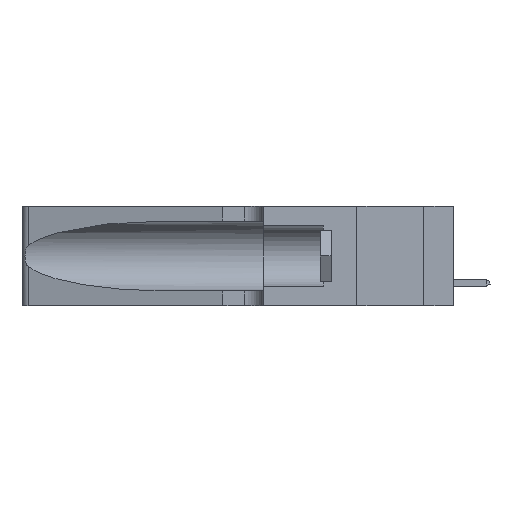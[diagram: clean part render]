
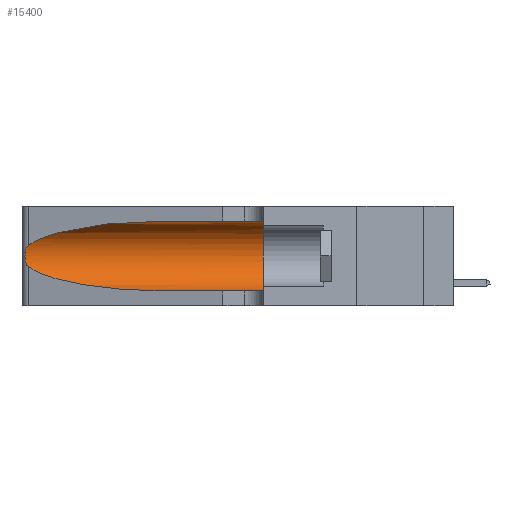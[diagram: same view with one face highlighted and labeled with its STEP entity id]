
A CAD part, left-side view. The second image highlights one B-rep face of the part: STEP entity #15400.
In plain terms, the highlighted cylindrical face has radius 3.308 mm (diameter 6.617 mm), a partial arc.
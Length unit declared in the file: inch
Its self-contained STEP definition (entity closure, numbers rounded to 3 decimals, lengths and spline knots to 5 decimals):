
#1205 = CARTESIAN_POINT ( 'NONE',  ( 0.25555, 1.22993, 0.14849 ) ) ;
#2419 = CARTESIAN_POINT ( 'NONE',  ( 0.1305, 1.61858, 0.05475 ) ) ;
#2559 = CARTESIAN_POINT ( 'NONE',  ( 0.25555, 1.22994, 0.2215 ) ) ;
#2878 = CARTESIAN_POINT ( 'NONE',  ( 0.1305, 0.35, 0.05475 ) ) ;
#3361 = EDGE_CURVE ( 'NONE', #26104, #41641, #37861, .T. ) ;
#3594 = CARTESIAN_POINT ( 'NONE',  ( 0.25639, 1.23184, 0.21858 ) ) ;
#3711 = ORIENTED_EDGE ( 'NONE', *, *, #20999, .T. ) ;
#3788 = CARTESIAN_POINT ( 'NONE',  ( 0.25854, 1.2359, 0.20912 ) ) ;
#4258 = DIRECTION ( 'NONE',  ( 0., -1., 0. ) ) ;
#4418 = CARTESIAN_POINT ( 'NONE',  ( 0.25487, 1.22718, 0.22369 ) ) ;
#4607 = CARTESIAN_POINT ( 'NONE',  ( 0.26075, 1.23896, 0.178 ) ) ;
#5104 = CARTESIAN_POINT ( 'NONE',  ( 0.26017, 1.23833, 0.17102 ) ) ;
#6530 =( BOUNDED_CURVE ( )  B_SPLINE_CURVE ( 3, ( #37726, #37422, #37571, #16501 ),
 .UNSPECIFIED., .F., .F. ) 
 B_SPLINE_CURVE_WITH_KNOTS ( ( 4, 4 ),
 ( 1.5708, 2.84003 ),
 .UNSPECIFIED. ) 
 CURVE ( )  GEOMETRIC_REPRESENTATION_ITEM ( )  RATIONAL_B_SPLINE_CURVE ( ( 1., 0.87, 0.87, 1. ) ) 
 REPRESENTATION_ITEM ( '' )  );
#10303 = CARTESIAN_POINT ( 'NONE',  ( 0.25856, 1.23593, 0.16098 ) ) ;
#10444 = CARTESIAN_POINT ( 'NONE',  ( 0.25639, 1.23186, 0.15144 ) ) ;
#12180 = EDGE_CURVE ( 'NONE', #22906, #26104, #22976, .T. ) ;
#13411 = VERTEX_POINT ( 'NONE', #21064 ) ;
#14017 = CARTESIAN_POINT ( 'NONE',  ( 0.25487, 1.22718, 0.14631 ) ) ;
#15400 = ADVANCED_FACE ( 'NONE', ( #46196 ), #45642, .F. ) ;
#15630 = ORIENTED_EDGE ( 'NONE', *, *, #21340, .T. ) ;
#16501 = CARTESIAN_POINT ( 'NONE',  ( 0.25487, 1.22718, 0.22369 ) ) ;
#16768 = ORIENTED_EDGE ( 'NONE', *, *, #12180, .F. ) ;
#18507 = CARTESIAN_POINT ( 'NONE',  ( 0.26018, 1.23835, 0.19895 ) ) ;
#19169 = CARTESIAN_POINT ( 'NONE',  ( 0.2373, 1.15595, 0.08982 ) ) ;
#20054 = CARTESIAN_POINT ( 'NONE',  ( 0.1305, 0.72297, 0.05475 ) ) ;
#20795 = DIRECTION ( 'NONE',  ( 0., -1., 0. ) ) ;
#20999 = EDGE_CURVE ( 'NONE', #25474, #33984, #41200, .T. ) ;
#21064 = CARTESIAN_POINT ( 'NONE',  ( 0.25487, 1.22718, 0.22369 ) ) ;
#21340 = EDGE_CURVE ( 'NONE', #13411, #25474, #46062, .T. ) ;
#21607 = CARTESIAN_POINT ( 'NONE',  ( 0.1305, 0.35, 0.185 ) ) ;
#21784 = EDGE_LOOP ( 'NONE', ( #43271, #15630, #3711, #34955, #45794, #16768 ) ) ;
#22006 = VECTOR ( 'NONE', #20795, 39.37008 ) ;
#22906 = VERTEX_POINT ( 'NONE', #33989 ) ;
#22976 = LINE ( 'NONE', #27740, #26335 ) ;
#23672 = CARTESIAN_POINT ( 'NONE',  ( 0.25787, 1.23484, 0.2124 ) ) ;
#25474 = VERTEX_POINT ( 'NONE', #29177 ) ;
#25748 = DIRECTION ( 'NONE',  ( 0., 0., 1. ) ) ;
#25834 = DIRECTION ( 'NONE',  ( 0., 0., -1. ) ) ;
#26016 = CARTESIAN_POINT ( 'NONE',  ( 0.18966, 0.96281, 0.05475 ) ) ;
#26104 = VERTEX_POINT ( 'NONE', #40741 ) ;
#26335 = VECTOR ( 'NONE', #30013, 39.37008 ) ;
#27740 = CARTESIAN_POINT ( 'NONE',  ( 0.1305, 1.61858, 0.31525 ) ) ;
#29007 = CARTESIAN_POINT ( 'NONE',  ( 0.1305, 1.61858, 0.185 ) ) ;
#29177 = CARTESIAN_POINT ( 'NONE',  ( 0.25487, 1.22718, 0.14631 ) ) ;
#29417 = EDGE_CURVE ( 'NONE', #33984, #41641, #30432, .T. ) ;
#29469 = CARTESIAN_POINT ( 'NONE',  ( 0.1305, 0.72297, 0.05475 ) ) ;
#30013 = DIRECTION ( 'NONE',  ( 0., -1., 0. ) ) ;
#30432 = LINE ( 'NONE', #2419, #22006 ) ;
#30737 = AXIS2_PLACEMENT_3D ( 'NONE', #29007, #4258, #25834 ) ;
#32545 = DIRECTION ( 'NONE',  ( 0., 1., 0. ) ) ;
#33984 = VERTEX_POINT ( 'NONE', #20054 ) ;
#33989 = CARTESIAN_POINT ( 'NONE',  ( 0.1305, 0.72297, 0.31525 ) ) ;
#34955 = ORIENTED_EDGE ( 'NONE', *, *, #29417, .T. ) ;
#37422 = CARTESIAN_POINT ( 'NONE',  ( 0.18966, 0.96281, 0.31525 ) ) ;
#37571 = CARTESIAN_POINT ( 'NONE',  ( 0.2373, 1.15595, 0.28018 ) ) ;
#37726 = CARTESIAN_POINT ( 'NONE',  ( 0.1305, 0.72297, 0.31525 ) ) ;
#37861 = CIRCLE ( 'NONE', #44473, 0.13025 ) ;
#40079 = CARTESIAN_POINT ( 'NONE',  ( 0.25487, 1.22718, 0.14631 ) ) ;
#40741 = CARTESIAN_POINT ( 'NONE',  ( 0.1305, 0.35, 0.31525 ) ) ;
#41200 =( BOUNDED_CURVE ( )  B_SPLINE_CURVE ( 3, ( #40079, #19169, #26016, #29469 ),
 .UNSPECIFIED., .F., .F. ) 
 B_SPLINE_CURVE_WITH_KNOTS ( ( 4, 4 ),
 ( 3.44316, 4.71239 ),
 .UNSPECIFIED. ) 
 CURVE ( )  GEOMETRIC_REPRESENTATION_ITEM ( )  RATIONAL_B_SPLINE_CURVE ( ( 1., 0.87, 0.87, 1. ) ) 
 REPRESENTATION_ITEM ( '' )  );
#41641 = VERTEX_POINT ( 'NONE', #2878 ) ;
#43271 = ORIENTED_EDGE ( 'NONE', *, *, #44158, .T. ) ;
#43517 = CARTESIAN_POINT ( 'NONE',  ( 0.26075, 1.23896, 0.19203 ) ) ;
#44158 = EDGE_CURVE ( 'NONE', #22906, #13411, #6530, .T. ) ;
#44473 = AXIS2_PLACEMENT_3D ( 'NONE', #21607, #32545, #25748 ) ;
#45642 = CYLINDRICAL_SURFACE ( 'NONE', #30737, 0.13025 ) ;
#45794 = ORIENTED_EDGE ( 'NONE', *, *, #3361, .F. ) ;
#46062 = B_SPLINE_CURVE_WITH_KNOTS ( 'NONE', 3,
 ( #4418, #2559, #3594, #23672, #3788, #18507, #43517, #4607, #5104, #10303, #46077, #10444, #1205, #14017 ),
 .UNSPECIFIED., .F., .F.,
 ( 4, 2, 2, 2, 2, 2, 4 ),
 ( 0., 0.00027, 0.00053, 0.00107, 0.0016, 0.00187, 0.00214 ),
 .UNSPECIFIED. ) ;
#46077 = CARTESIAN_POINT ( 'NONE',  ( 0.25789, 1.23486, 0.15765 ) ) ;
#46196 = FACE_OUTER_BOUND ( 'NONE', #21784, .T. ) ;
